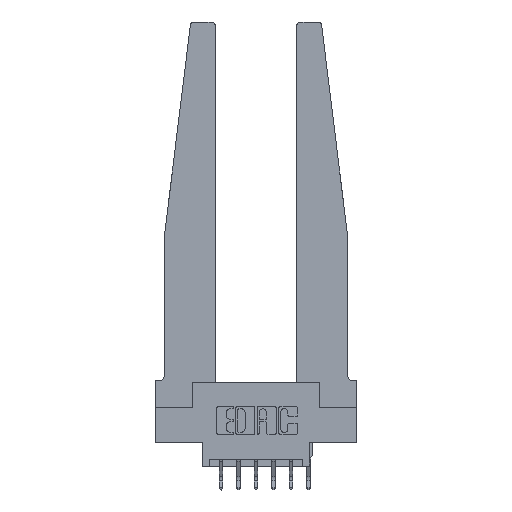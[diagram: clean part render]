
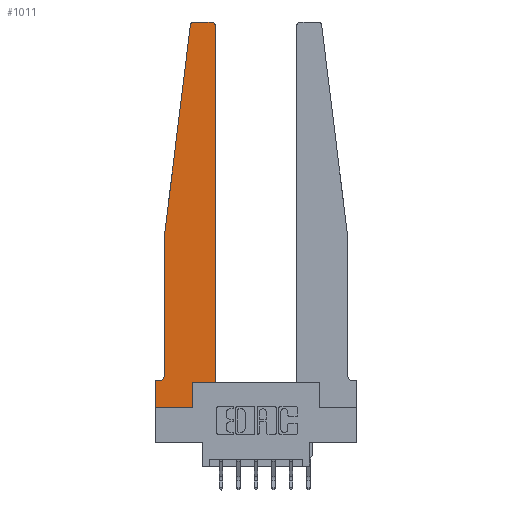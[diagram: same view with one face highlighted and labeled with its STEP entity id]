
A CAD part, top view. The second image highlights one B-rep face of the part: STEP entity #1011.
In plain terms, the highlighted planar face has unit normal (0, 0, 1).
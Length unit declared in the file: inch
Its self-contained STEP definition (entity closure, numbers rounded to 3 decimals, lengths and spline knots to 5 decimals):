
#6 = DIRECTION ( 'NONE',  ( 0., 0., 1. ) ) ;
#132 = LINE ( 'NONE', #3334, #11949 ) ;
#221 = LINE ( 'NONE', #10941, #8677 ) ;
#384 = VECTOR ( 'NONE', #4765, 39.37008 ) ;
#437 = VERTEX_POINT ( 'NONE', #3265 ) ;
#581 = LINE ( 'NONE', #11279, #8003 ) ;
#598 = VERTEX_POINT ( 'NONE', #2061 ) ;
#1011 = ADVANCED_FACE ( 'NONE', ( #7428 ), #4203, .T. ) ;
#1070 = CARTESIAN_POINT ( 'NONE',  ( 0.015, 0.2375, 0.37 ) ) ;
#1395 = ORIENTED_EDGE ( 'NONE', *, *, #9094, .T. ) ;
#1419 = AXIS2_PLACEMENT_3D ( 'NONE', #9543, #6, #3216 ) ;
#2061 = CARTESIAN_POINT ( 'NONE',  ( 0.425, 0.18, 0.37 ) ) ;
#2073 = AXIS2_PLACEMENT_3D ( 'NONE', #1070, #4544, #4269 ) ;
#2184 = CARTESIAN_POINT ( 'NONE',  ( 0.065, 1.25, 0.37 ) ) ;
#2870 = DIRECTION ( 'NONE',  ( 1., 0., 0. ) ) ;
#2934 = CARTESIAN_POINT ( 'NONE',  ( 0.2605, 0., 0.37 ) ) ;
#3072 = DIRECTION ( 'NONE',  ( 1., 0., 0. ) ) ;
#3216 = DIRECTION ( 'NONE',  ( 1., 0., 0. ) ) ;
#3265 = CARTESIAN_POINT ( 'NONE',  ( 0.425, 2.72, 0.37 ) ) ;
#3334 = CARTESIAN_POINT ( 'NONE',  ( 0.065, 1.25, 0.37 ) ) ;
#3365 = CARTESIAN_POINT ( 'NONE',  ( 0.2605, 0.18, 0.37 ) ) ;
#3379 = CARTESIAN_POINT ( 'NONE',  ( 0.425, 0.18, 0.37 ) ) ;
#3397 = DIRECTION ( 'NONE',  ( -0.122, -0.992, 0. ) ) ;
#3483 = CARTESIAN_POINT ( 'NONE',  ( 0.27653, 2.75, 0.37 ) ) ;
#3569 = DIRECTION ( 'NONE',  ( 0., -1., 0. ) ) ;
#3661 = CIRCLE ( 'NONE', #6796, 0.03 ) ;
#3964 = CARTESIAN_POINT ( 'NONE',  ( 0.015, 0.1875, 0.37 ) ) ;
#4115 = LINE ( 'NONE', #8533, #6631 ) ;
#4203 = PLANE ( 'NONE',  #1419 ) ;
#4209 = VERTEX_POINT ( 'NONE', #3483 ) ;
#4269 = DIRECTION ( 'NONE',  ( -1., 0., 0. ) ) ;
#4514 = EDGE_CURVE ( 'NONE', #6649, #11909, #9785, .T. ) ;
#4544 = DIRECTION ( 'NONE',  ( 0., 0., -1. ) ) ;
#4673 = EDGE_CURVE ( 'NONE', #13516, #5892, #12283, .T. ) ;
#4765 = DIRECTION ( 'NONE',  ( 0., -1., 0. ) ) ;
#5184 = ORIENTED_EDGE ( 'NONE', *, *, #5378, .T. ) ;
#5207 = CIRCLE ( 'NONE', #2073, 0.05 ) ;
#5219 = CARTESIAN_POINT ( 'NONE',  ( 0., 0., 0.37 ) ) ;
#5378 = EDGE_CURVE ( 'NONE', #5892, #6649, #4115, .T. ) ;
#5634 = CARTESIAN_POINT ( 'NONE',  ( 0.395, 2.75, 0.37 ) ) ;
#5786 = ORIENTED_EDGE ( 'NONE', *, *, #10192, .T. ) ;
#5795 = DIRECTION ( 'NONE',  ( 1., 0., 0. ) ) ;
#5860 = VECTOR ( 'NONE', #10776, 39.37008 ) ;
#5875 = EDGE_CURVE ( 'NONE', #437, #9239, #10013, .T. ) ;
#5892 = VERTEX_POINT ( 'NONE', #5219 ) ;
#5906 = CARTESIAN_POINT ( 'NONE',  ( 0.24675, 2.72367, 0.37 ) ) ;
#5957 = ORIENTED_EDGE ( 'NONE', *, *, #8286, .T. ) ;
#5996 = ORIENTED_EDGE ( 'NONE', *, *, #6658, .T. ) ;
#6038 = CARTESIAN_POINT ( 'NONE',  ( 0.065, 0.1875, 0.37 ) ) ;
#6351 = LINE ( 'NONE', #10648, #5860 ) ;
#6400 = DIRECTION ( 'NONE',  ( 0., 1., 0. ) ) ;
#6510 = EDGE_CURVE ( 'NONE', #13119, #10102, #221, .T. ) ;
#6631 = VECTOR ( 'NONE', #3072, 39.37008 ) ;
#6641 = ORIENTED_EDGE ( 'NONE', *, *, #5875, .T. ) ;
#6649 = VERTEX_POINT ( 'NONE', #2934 ) ;
#6658 = EDGE_CURVE ( 'NONE', #11909, #598, #581, .T. ) ;
#6776 = VECTOR ( 'NONE', #6400, 39.37008 ) ;
#6796 = AXIS2_PLACEMENT_3D ( 'NONE', #6854, #11136, #5795 ) ;
#6854 = CARTESIAN_POINT ( 'NONE',  ( 0.27653, 2.72, 0.37 ) ) ;
#6952 = CARTESIAN_POINT ( 'NONE',  ( 0.2605, 0.18, 0.37 ) ) ;
#7057 = ORIENTED_EDGE ( 'NONE', *, *, #12850, .T. ) ;
#7428 = FACE_OUTER_BOUND ( 'NONE', #9195, .T. ) ;
#7652 = DIRECTION ( 'NONE',  ( 0., 1., 0. ) ) ;
#7843 = CARTESIAN_POINT ( 'NONE',  ( 0.065, 0.2375, 0.37 ) ) ;
#8003 = VECTOR ( 'NONE', #2870, 39.37008 ) ;
#8286 = EDGE_CURVE ( 'NONE', #598, #437, #13004, .T. ) ;
#8533 = CARTESIAN_POINT ( 'NONE',  ( 0., 0., 0.37 ) ) ;
#8574 = EDGE_CURVE ( 'NONE', #11767, #13516, #11374, .T. ) ;
#8677 = VECTOR ( 'NONE', #3569, 39.37008 ) ;
#9094 = EDGE_CURVE ( 'NONE', #11898, #13119, #132, .T. ) ;
#9195 = EDGE_LOOP ( 'NONE', ( #7057, #5786, #1395, #13754, #13681, #10621, #11019, #5184, #11320, #5996, #5957, #6641 ) ) ;
#9239 = VERTEX_POINT ( 'NONE', #5634 ) ;
#9484 = VECTOR ( 'NONE', #10411, 39.37008 ) ;
#9543 = CARTESIAN_POINT ( 'NONE',  ( 0., 0.1875, 0.37 ) ) ;
#9585 = DIRECTION ( 'NONE',  ( 0., 0., 1. ) ) ;
#9785 = LINE ( 'NONE', #3365, #13352 ) ;
#9908 = CARTESIAN_POINT ( 'NONE',  ( 0., 0., 0.37 ) ) ;
#10013 = CIRCLE ( 'NONE', #11123, 0.03 ) ;
#10102 = VERTEX_POINT ( 'NONE', #7843 ) ;
#10192 = EDGE_CURVE ( 'NONE', #4209, #11898, #3661, .T. ) ;
#10411 = DIRECTION ( 'NONE',  ( -1., 0., 0. ) ) ;
#10621 = ORIENTED_EDGE ( 'NONE', *, *, #8574, .T. ) ;
#10648 = CARTESIAN_POINT ( 'NONE',  ( 0.25, 2.75, 0.37 ) ) ;
#10776 = DIRECTION ( 'NONE',  ( -1., 0., 0. ) ) ;
#10941 = CARTESIAN_POINT ( 'NONE',  ( 0.065, 1.25, 0.37 ) ) ;
#11019 = ORIENTED_EDGE ( 'NONE', *, *, #4673, .T. ) ;
#11123 = AXIS2_PLACEMENT_3D ( 'NONE', #12806, #9585, #13868 ) ;
#11136 = DIRECTION ( 'NONE',  ( 0., 0., 1. ) ) ;
#11279 = CARTESIAN_POINT ( 'NONE',  ( 0.425, 0.18, 0.37 ) ) ;
#11320 = ORIENTED_EDGE ( 'NONE', *, *, #4514, .T. ) ;
#11374 = LINE ( 'NONE', #6038, #9484 ) ;
#11767 = VERTEX_POINT ( 'NONE', #3964 ) ;
#11898 = VERTEX_POINT ( 'NONE', #5906 ) ;
#11909 = VERTEX_POINT ( 'NONE', #6952 ) ;
#11949 = VECTOR ( 'NONE', #3397, 39.37008 ) ;
#12283 = LINE ( 'NONE', #9908, #384 ) ;
#12806 = CARTESIAN_POINT ( 'NONE',  ( 0.395, 2.72, 0.37 ) ) ;
#12839 = CARTESIAN_POINT ( 'NONE',  ( 0., 0.1875, 0.37 ) ) ;
#12850 = EDGE_CURVE ( 'NONE', #9239, #4209, #6351, .T. ) ;
#13004 = LINE ( 'NONE', #3379, #6776 ) ;
#13119 = VERTEX_POINT ( 'NONE', #2184 ) ;
#13352 = VECTOR ( 'NONE', #7652, 39.37008 ) ;
#13516 = VERTEX_POINT ( 'NONE', #12839 ) ;
#13517 = EDGE_CURVE ( 'NONE', #10102, #11767, #5207, .T. ) ;
#13681 = ORIENTED_EDGE ( 'NONE', *, *, #13517, .T. ) ;
#13754 = ORIENTED_EDGE ( 'NONE', *, *, #6510, .T. ) ;
#13868 = DIRECTION ( 'NONE',  ( 1., 0., 0. ) ) ;
